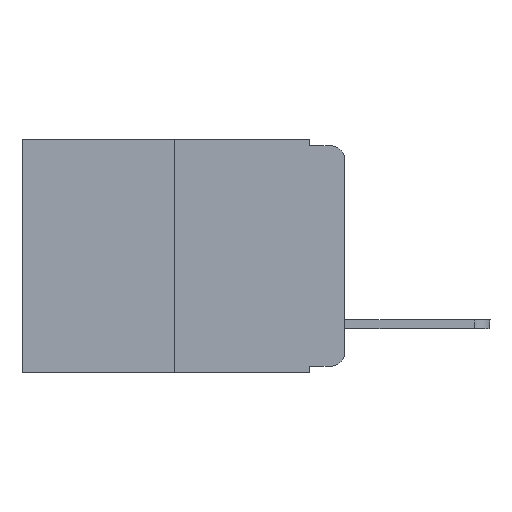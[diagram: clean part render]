
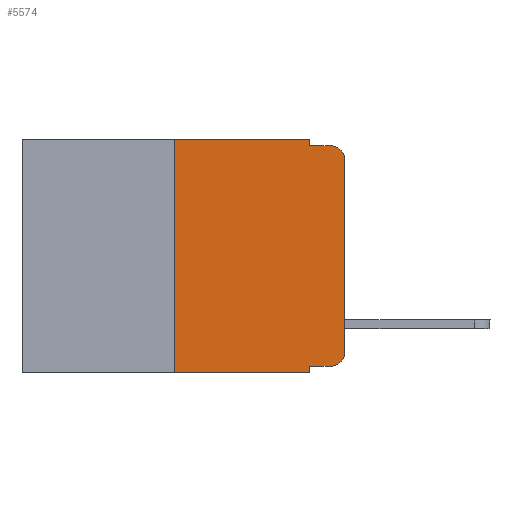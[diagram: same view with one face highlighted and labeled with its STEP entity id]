
A CAD part, left-side view. The second image highlights one B-rep face of the part: STEP entity #5574.
In plain terms, the highlighted planar face has unit normal (-1, 0, 0).
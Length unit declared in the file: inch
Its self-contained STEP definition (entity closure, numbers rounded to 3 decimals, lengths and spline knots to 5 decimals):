
#26 = VERTEX_POINT ( 'NONE', #11745 ) ;
#271 = ORIENTED_EDGE ( 'NONE', *, *, #6158, .F. ) ;
#286 = CARTESIAN_POINT ( 'NONE',  ( 0., 0.473, 0. ) ) ;
#905 = ORIENTED_EDGE ( 'NONE', *, *, #4265, .F. ) ;
#923 = CARTESIAN_POINT ( 'NONE',  ( 0., 0., -0.313 ) ) ;
#1087 = DIRECTION ( 'NONE',  ( 0., -1., 0. ) ) ;
#1089 = CARTESIAN_POINT ( 'NONE',  ( 0., 0.02, -0.03 ) ) ;
#1120 = LINE ( 'NONE', #3700, #7307 ) ;
#1469 = LINE ( 'NONE', #5728, #13888 ) ;
#1605 = EDGE_CURVE ( 'NONE', #2445, #13650, #1985, .T. ) ;
#1680 = CARTESIAN_POINT ( 'NONE',  ( 0., 0.051, 0. ) ) ;
#1716 = CARTESIAN_POINT ( 'NONE',  ( 0., 0., 0. ) ) ;
#1820 = CARTESIAN_POINT ( 'NONE',  ( 0., 0.051, -0.333 ) ) ;
#1921 = LINE ( 'NONE', #11575, #15139 ) ;
#1985 = LINE ( 'NONE', #5307, #10981 ) ;
#2445 = VERTEX_POINT ( 'NONE', #3230 ) ;
#2518 = EDGE_CURVE ( 'NONE', #4601, #13650, #5538, .T. ) ;
#2663 = VERTEX_POINT ( 'NONE', #8954 ) ;
#3127 = LINE ( 'NONE', #4918, #12760 ) ;
#3230 = CARTESIAN_POINT ( 'NONE',  ( 0., 0.051, -0.01 ) ) ;
#3283 = DIRECTION ( 'NONE',  ( 0., 0., -1. ) ) ;
#3333 = VECTOR ( 'NONE', #8288, 39.37008 ) ;
#3593 = ORIENTED_EDGE ( 'NONE', *, *, #4434, .T. ) ;
#3677 = ORIENTED_EDGE ( 'NONE', *, *, #10102, .T. ) ;
#3700 = CARTESIAN_POINT ( 'NONE',  ( 0., 0.25, 0. ) ) ;
#3787 = VERTEX_POINT ( 'NONE', #1820 ) ;
#4038 = EDGE_LOOP ( 'NONE', ( #14547, #5046, #11796, #271, #8010, #905, #3593, #8674, #3677, #16053 ) ) ;
#4265 = EDGE_CURVE ( 'NONE', #26, #10297, #1120, .T. ) ;
#4312 = DIRECTION ( 'NONE',  ( 0., 0., 1. ) ) ;
#4406 = AXIS2_PLACEMENT_3D ( 'NONE', #8461, #7270, #3283 ) ;
#4434 = EDGE_CURVE ( 'NONE', #26, #4511, #1921, .T. ) ;
#4511 = VERTEX_POINT ( 'NONE', #11803 ) ;
#4601 = VERTEX_POINT ( 'NONE', #5461 ) ;
#4918 = CARTESIAN_POINT ( 'NONE',  ( 0., 0.051, -0.333 ) ) ;
#5046 = ORIENTED_EDGE ( 'NONE', *, *, #2518, .T. ) ;
#5307 = CARTESIAN_POINT ( 'NONE',  ( 0., 0.051, -0.01 ) ) ;
#5435 = CIRCLE ( 'NONE', #9532, 0.02 ) ;
#5461 = CARTESIAN_POINT ( 'NONE',  ( 0., 0., -0.03 ) ) ;
#5538 = CIRCLE ( 'NONE', #8432, 0.02 ) ;
#5574 = ADVANCED_FACE ( 'NONE', ( #10058 ), #11001, .F. ) ;
#5728 = CARTESIAN_POINT ( 'NONE',  ( 0., 0.051, 0. ) ) ;
#6158 = EDGE_CURVE ( 'NONE', #8576, #2445, #1469, .T. ) ;
#7042 = CARTESIAN_POINT ( 'NONE',  ( 0., 0.051, 0. ) ) ;
#7270 = DIRECTION ( 'NONE',  ( 1., 0., 0. ) ) ;
#7307 = VECTOR ( 'NONE', #15180, 39.37008 ) ;
#8010 = ORIENTED_EDGE ( 'NONE', *, *, #8560, .F. ) ;
#8288 = DIRECTION ( 'NONE',  ( 0., 0., -1. ) ) ;
#8432 = AXIS2_PLACEMENT_3D ( 'NONE', #1089, #11180, #9993 ) ;
#8461 = CARTESIAN_POINT ( 'NONE',  ( 0., 0.473, 0. ) ) ;
#8560 = EDGE_CURVE ( 'NONE', #10297, #8576, #9113, .T. ) ;
#8576 = VERTEX_POINT ( 'NONE', #1680 ) ;
#8674 = ORIENTED_EDGE ( 'NONE', *, *, #12582, .F. ) ;
#8954 = CARTESIAN_POINT ( 'NONE',  ( 0., 0.02, -0.333 ) ) ;
#9113 = LINE ( 'NONE', #286, #10345 ) ;
#9167 = EDGE_CURVE ( 'NONE', #15951, #4601, #15777, .T. ) ;
#9511 = CARTESIAN_POINT ( 'NONE',  ( 0., 0.02, -0.313 ) ) ;
#9532 = AXIS2_PLACEMENT_3D ( 'NONE', #9511, #11844, #10652 ) ;
#9993 = DIRECTION ( 'NONE',  ( 0., 0., -1. ) ) ;
#10058 = FACE_OUTER_BOUND ( 'NONE', #4038, .T. ) ;
#10102 = EDGE_CURVE ( 'NONE', #3787, #2663, #3127, .T. ) ;
#10297 = VERTEX_POINT ( 'NONE', #12824 ) ;
#10345 = VECTOR ( 'NONE', #10668, 39.37008 ) ;
#10652 = DIRECTION ( 'NONE',  ( 0., 0., -1. ) ) ;
#10668 = DIRECTION ( 'NONE',  ( 0., -1., 0. ) ) ;
#10981 = VECTOR ( 'NONE', #14467, 39.37008 ) ;
#10984 = DIRECTION ( 'NONE',  ( 0., 0., -1. ) ) ;
#11001 = PLANE ( 'NONE',  #4406 ) ;
#11180 = DIRECTION ( 'NONE',  ( -1., 0., 0. ) ) ;
#11575 = CARTESIAN_POINT ( 'NONE',  ( 0., 0.473, -0.343 ) ) ;
#11745 = CARTESIAN_POINT ( 'NONE',  ( 0., 0.25, -0.343 ) ) ;
#11796 = ORIENTED_EDGE ( 'NONE', *, *, #1605, .F. ) ;
#11803 = CARTESIAN_POINT ( 'NONE',  ( 0., 0.051, -0.343 ) ) ;
#11844 = DIRECTION ( 'NONE',  ( -1., 0., 0. ) ) ;
#12165 = LINE ( 'NONE', #7042, #3333 ) ;
#12582 = EDGE_CURVE ( 'NONE', #3787, #4511, #12165, .T. ) ;
#12760 = VECTOR ( 'NONE', #1087, 39.37008 ) ;
#12824 = CARTESIAN_POINT ( 'NONE',  ( 0., 0.25, 0. ) ) ;
#13650 = VERTEX_POINT ( 'NONE', #14204 ) ;
#13888 = VECTOR ( 'NONE', #10984, 39.37008 ) ;
#14204 = CARTESIAN_POINT ( 'NONE',  ( 0., 0.02, -0.01 ) ) ;
#14353 = DIRECTION ( 'NONE',  ( 0., -1., 0. ) ) ;
#14467 = DIRECTION ( 'NONE',  ( 0., -1., 0. ) ) ;
#14547 = ORIENTED_EDGE ( 'NONE', *, *, #9167, .T. ) ;
#14964 = VECTOR ( 'NONE', #4312, 39.37008 ) ;
#15139 = VECTOR ( 'NONE', #14353, 39.37008 ) ;
#15180 = DIRECTION ( 'NONE',  ( 0., 0., 1. ) ) ;
#15181 = EDGE_CURVE ( 'NONE', #2663, #15951, #5435, .T. ) ;
#15777 = LINE ( 'NONE', #1716, #14964 ) ;
#15951 = VERTEX_POINT ( 'NONE', #923 ) ;
#16053 = ORIENTED_EDGE ( 'NONE', *, *, #15181, .T. ) ;
